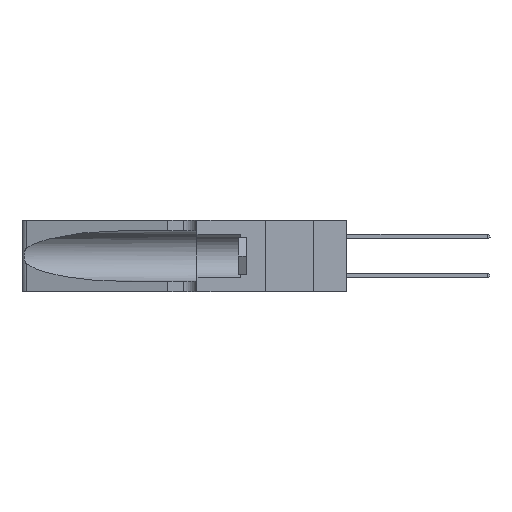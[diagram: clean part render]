
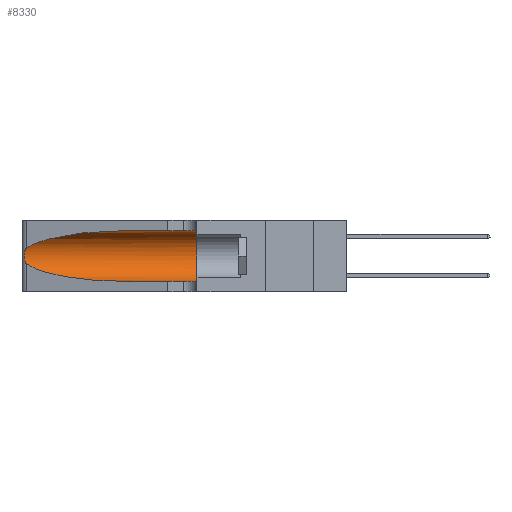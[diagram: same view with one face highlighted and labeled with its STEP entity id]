
A CAD part, left-side view. The second image highlights one B-rep face of the part: STEP entity #8330.
In plain terms, the highlighted cylindrical face has radius 3.308 mm (diameter 6.617 mm), a partial arc.
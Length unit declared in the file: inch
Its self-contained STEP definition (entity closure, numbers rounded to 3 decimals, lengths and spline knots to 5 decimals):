
#108 = CARTESIAN_POINT ( 'NONE',  ( 0.26017, 1.23833, 0.17102 ) ) ;
#284 = B_SPLINE_CURVE_WITH_KNOTS ( 'NONE', 3,
 ( #6317, #7319, #2725, #9909, #21278, #6273, #9938, #14725, #108, #7488, #8979, #22960, #22583, #17091 ),
 .UNSPECIFIED., .F., .F.,
 ( 4, 2, 2, 2, 2, 2, 4 ),
 ( 0., 0.00027, 0.00053, 0.00107, 0.0016, 0.00187, 0.00214 ),
 .UNSPECIFIED. ) ;
#330 = CARTESIAN_POINT ( 'NONE',  ( 0.1305, 0.35, 0.31525 ) ) ;
#439 = CARTESIAN_POINT ( 'NONE',  ( 0.1305, 1.61858, 0.185 ) ) ;
#761 = CARTESIAN_POINT ( 'NONE',  ( 0.1305, 0.35, 0.05475 ) ) ;
#1156 = EDGE_CURVE ( 'NONE', #5664, #14188, #284, .T. ) ;
#1591 = ORIENTED_EDGE ( 'NONE', *, *, #13911, .T. ) ;
#1674 = CARTESIAN_POINT ( 'NONE',  ( 0.25487, 1.22718, 0.22369 ) ) ;
#2044 = CARTESIAN_POINT ( 'NONE',  ( 0.1305, 0.72297, 0.05475 ) ) ;
#2367 = DIRECTION ( 'NONE',  ( 0., 0., -1. ) ) ;
#2725 = CARTESIAN_POINT ( 'NONE',  ( 0.25639, 1.23184, 0.21858 ) ) ;
#2726 = ORIENTED_EDGE ( 'NONE', *, *, #1156, .T. ) ;
#2763 = VECTOR ( 'NONE', #17950, 39.37008 ) ;
#3990 = AXIS2_PLACEMENT_3D ( 'NONE', #5673, #18640, #7587 ) ;
#4251 = EDGE_CURVE ( 'NONE', #8804, #5669, #16155, .T. ) ;
#5664 = VERTEX_POINT ( 'NONE', #8290 ) ;
#5669 = VERTEX_POINT ( 'NONE', #761 ) ;
#5673 = CARTESIAN_POINT ( 'NONE',  ( 0.1305, 0.35, 0.185 ) ) ;
#5756 = CARTESIAN_POINT ( 'NONE',  ( 0.25487, 1.22718, 0.14631 ) ) ;
#6273 = CARTESIAN_POINT ( 'NONE',  ( 0.26018, 1.23835, 0.19895 ) ) ;
#6317 = CARTESIAN_POINT ( 'NONE',  ( 0.25487, 1.22718, 0.22369 ) ) ;
#6654 = ORIENTED_EDGE ( 'NONE', *, *, #10801, .T. ) ;
#7319 = CARTESIAN_POINT ( 'NONE',  ( 0.25555, 1.22994, 0.2215 ) ) ;
#7488 = CARTESIAN_POINT ( 'NONE',  ( 0.25856, 1.23593, 0.16098 ) ) ;
#7587 = DIRECTION ( 'NONE',  ( 0., 0., 1. ) ) ;
#7644 = CARTESIAN_POINT ( 'NONE',  ( 0.2373, 1.15595, 0.08982 ) ) ;
#7935 =( BOUNDED_CURVE ( )  B_SPLINE_CURVE ( 3, ( #15042, #7644, #13294, #2044 ),
 .UNSPECIFIED., .F., .T. ) 
 B_SPLINE_CURVE_WITH_KNOTS ( ( 4, 4 ),
 ( 3.44316, 4.71239 ),
 .UNSPECIFIED. ) 
 CURVE ( )  GEOMETRIC_REPRESENTATION_ITEM ( )  RATIONAL_B_SPLINE_CURVE ( ( 1., 0.87, 0.87, 1. ) ) 
 REPRESENTATION_ITEM ( '' )  );
#7982 = DIRECTION ( 'NONE',  ( 0., -1., 0. ) ) ;
#8290 = CARTESIAN_POINT ( 'NONE',  ( 0.25487, 1.22718, 0.22369 ) ) ;
#8330 = ADVANCED_FACE ( 'NONE', ( #11422 ), #20543, .F. ) ;
#8780 = CARTESIAN_POINT ( 'NONE',  ( 0.1305, 1.61858, 0.05475 ) ) ;
#8804 = VERTEX_POINT ( 'NONE', #330 ) ;
#8979 = CARTESIAN_POINT ( 'NONE',  ( 0.25789, 1.23486, 0.15765 ) ) ;
#9909 = CARTESIAN_POINT ( 'NONE',  ( 0.25787, 1.23484, 0.2124 ) ) ;
#9938 = CARTESIAN_POINT ( 'NONE',  ( 0.26075, 1.23896, 0.19203 ) ) ;
#10199 = VERTEX_POINT ( 'NONE', #14614 ) ;
#10294 = EDGE_LOOP ( 'NONE', ( #6654, #2726, #15003, #1591, #16262, #11145 ) ) ;
#10801 = EDGE_CURVE ( 'NONE', #10199, #5664, #13140, .T. ) ;
#11076 = CARTESIAN_POINT ( 'NONE',  ( 0.1305, 0.72297, 0.31525 ) ) ;
#11145 = ORIENTED_EDGE ( 'NONE', *, *, #17731, .F. ) ;
#11422 = FACE_OUTER_BOUND ( 'NONE', #10294, .T. ) ;
#11776 = CARTESIAN_POINT ( 'NONE',  ( 0.1305, 1.61858, 0.31525 ) ) ;
#12666 = VECTOR ( 'NONE', #22683, 39.37008 ) ;
#12940 = CARTESIAN_POINT ( 'NONE',  ( 0.2373, 1.15595, 0.28018 ) ) ;
#13140 =( BOUNDED_CURVE ( )  B_SPLINE_CURVE ( 3, ( #11076, #18335, #12940, #1674 ),
 .UNSPECIFIED., .F., .F. ) 
 B_SPLINE_CURVE_WITH_KNOTS ( ( 4, 4 ),
 ( 1.5708, 2.84003 ),
 .UNSPECIFIED. ) 
 CURVE ( )  GEOMETRIC_REPRESENTATION_ITEM ( )  RATIONAL_B_SPLINE_CURVE ( ( 1., 0.87, 0.87, 1. ) ) 
 REPRESENTATION_ITEM ( '' )  );
#13294 = CARTESIAN_POINT ( 'NONE',  ( 0.18966, 0.96281, 0.05475 ) ) ;
#13911 = EDGE_CURVE ( 'NONE', #20927, #5669, #22450, .T. ) ;
#14188 = VERTEX_POINT ( 'NONE', #5756 ) ;
#14614 = CARTESIAN_POINT ( 'NONE',  ( 0.1305, 0.72297, 0.31525 ) ) ;
#14725 = CARTESIAN_POINT ( 'NONE',  ( 0.26075, 1.23896, 0.178 ) ) ;
#15003 = ORIENTED_EDGE ( 'NONE', *, *, #17637, .T. ) ;
#15042 = CARTESIAN_POINT ( 'NONE',  ( 0.25487, 1.22718, 0.14631 ) ) ;
#16155 = CIRCLE ( 'NONE', #3990, 0.13025 ) ;
#16262 = ORIENTED_EDGE ( 'NONE', *, *, #4251, .F. ) ;
#17091 = CARTESIAN_POINT ( 'NONE',  ( 0.25487, 1.22718, 0.14631 ) ) ;
#17481 = LINE ( 'NONE', #11776, #12666 ) ;
#17605 = AXIS2_PLACEMENT_3D ( 'NONE', #439, #7982, #2367 ) ;
#17637 = EDGE_CURVE ( 'NONE', #14188, #20927, #7935, .T. ) ;
#17731 = EDGE_CURVE ( 'NONE', #10199, #8804, #17481, .T. ) ;
#17950 = DIRECTION ( 'NONE',  ( 0., -1., 0. ) ) ;
#18335 = CARTESIAN_POINT ( 'NONE',  ( 0.18966, 0.96281, 0.31525 ) ) ;
#18640 = DIRECTION ( 'NONE',  ( 0., 1., 0. ) ) ;
#20543 = CYLINDRICAL_SURFACE ( 'NONE', #17605, 0.13025 ) ;
#20927 = VERTEX_POINT ( 'NONE', #22737 ) ;
#21278 = CARTESIAN_POINT ( 'NONE',  ( 0.25854, 1.2359, 0.20912 ) ) ;
#22450 = LINE ( 'NONE', #8780, #2763 ) ;
#22583 = CARTESIAN_POINT ( 'NONE',  ( 0.25555, 1.22993, 0.14849 ) ) ;
#22683 = DIRECTION ( 'NONE',  ( 0., -1., 0. ) ) ;
#22737 = CARTESIAN_POINT ( 'NONE',  ( 0.1305, 0.72297, 0.05475 ) ) ;
#22960 = CARTESIAN_POINT ( 'NONE',  ( 0.25639, 1.23186, 0.15144 ) ) ;
